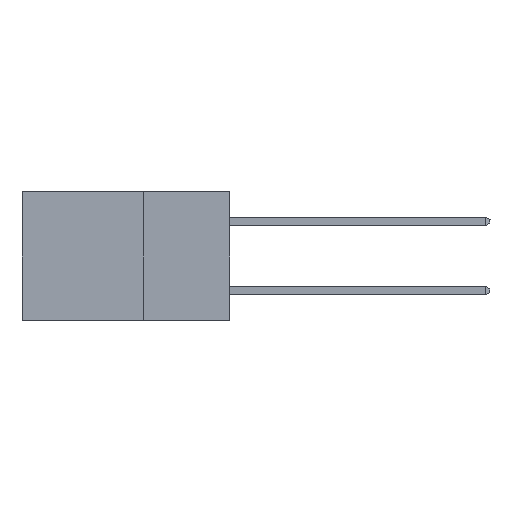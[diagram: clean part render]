
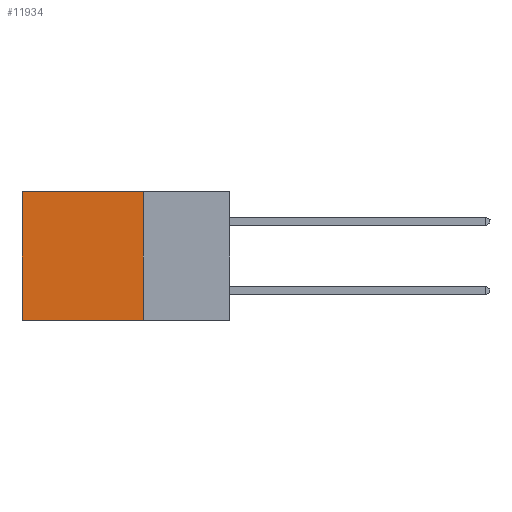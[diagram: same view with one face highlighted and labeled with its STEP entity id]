
A CAD part, left-side view. The second image highlights one B-rep face of the part: STEP entity #11934.
In plain terms, the highlighted planar face has unit normal (-1, 0, 0).
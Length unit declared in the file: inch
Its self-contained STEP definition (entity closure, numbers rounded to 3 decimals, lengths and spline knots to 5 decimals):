
#1448 = VECTOR ( 'NONE', #4686, 39.37008 ) ;
#2111 = PLANE ( 'NONE',  #10238 ) ;
#2541 = EDGE_CURVE ( 'NONE', #5128, #2833, #9203, .T. ) ;
#2677 = CARTESIAN_POINT ( 'NONE',  ( 0.2615, 0.25, 0. ) ) ;
#2773 = VECTOR ( 'NONE', #7465, 39.37008 ) ;
#2833 = VERTEX_POINT ( 'NONE', #10990 ) ;
#3028 = CARTESIAN_POINT ( 'NONE',  ( 0.2615, 0.25, -0.37 ) ) ;
#3110 = DIRECTION ( 'NONE',  ( 1., 0., 0. ) ) ;
#3631 = EDGE_CURVE ( 'NONE', #7769, #2833, #9830, .T. ) ;
#3715 = LINE ( 'NONE', #7595, #2773 ) ;
#3829 = EDGE_CURVE ( 'NONE', #6357, #5128, #10265, .T. ) ;
#4686 = DIRECTION ( 'NONE',  ( 0., 0., -1. ) ) ;
#5128 = VERTEX_POINT ( 'NONE', #3028 ) ;
#5605 = EDGE_LOOP ( 'NONE', ( #10151, #9581, #9990, #6607 ) ) ;
#6001 = VECTOR ( 'NONE', #11010, 39.37008 ) ;
#6357 = VERTEX_POINT ( 'NONE', #2677 ) ;
#6607 = ORIENTED_EDGE ( 'NONE', *, *, #11034, .T. ) ;
#6624 = FACE_OUTER_BOUND ( 'NONE', #5605, .T. ) ;
#6737 = CARTESIAN_POINT ( 'NONE',  ( 0.2615, 0.25, -0.37 ) ) ;
#7465 = DIRECTION ( 'NONE',  ( 0., 1., 0. ) ) ;
#7595 = CARTESIAN_POINT ( 'NONE',  ( 0.2615, 0.25, 0. ) ) ;
#7769 = VERTEX_POINT ( 'NONE', #11083 ) ;
#9022 = VECTOR ( 'NONE', #11944, 39.37008 ) ;
#9203 = LINE ( 'NONE', #12126, #6001 ) ;
#9338 = CARTESIAN_POINT ( 'NONE',  ( 0.2615, 0.25, -0.37 ) ) ;
#9581 = ORIENTED_EDGE ( 'NONE', *, *, #2541, .F. ) ;
#9604 = DIRECTION ( 'NONE',  ( 0., 0., -1. ) ) ;
#9830 = LINE ( 'NONE', #10950, #9022 ) ;
#9990 = ORIENTED_EDGE ( 'NONE', *, *, #3829, .F. ) ;
#10151 = ORIENTED_EDGE ( 'NONE', *, *, #3631, .T. ) ;
#10238 = AXIS2_PLACEMENT_3D ( 'NONE', #6737, #3110, #9604 ) ;
#10265 = LINE ( 'NONE', #9338, #1448 ) ;
#10950 = CARTESIAN_POINT ( 'NONE',  ( 0.2615, 0.6, -0.37 ) ) ;
#10990 = CARTESIAN_POINT ( 'NONE',  ( 0.2615, 0.6, -0.37 ) ) ;
#11010 = DIRECTION ( 'NONE',  ( 0., 1., 0. ) ) ;
#11034 = EDGE_CURVE ( 'NONE', #6357, #7769, #3715, .T. ) ;
#11083 = CARTESIAN_POINT ( 'NONE',  ( 0.2615, 0.6, 0. ) ) ;
#11934 = ADVANCED_FACE ( 'NONE', ( #6624 ), #2111, .F. ) ;
#11944 = DIRECTION ( 'NONE',  ( 0., 0., -1. ) ) ;
#12126 = CARTESIAN_POINT ( 'NONE',  ( 0.2615, 0.25, -0.37 ) ) ;
